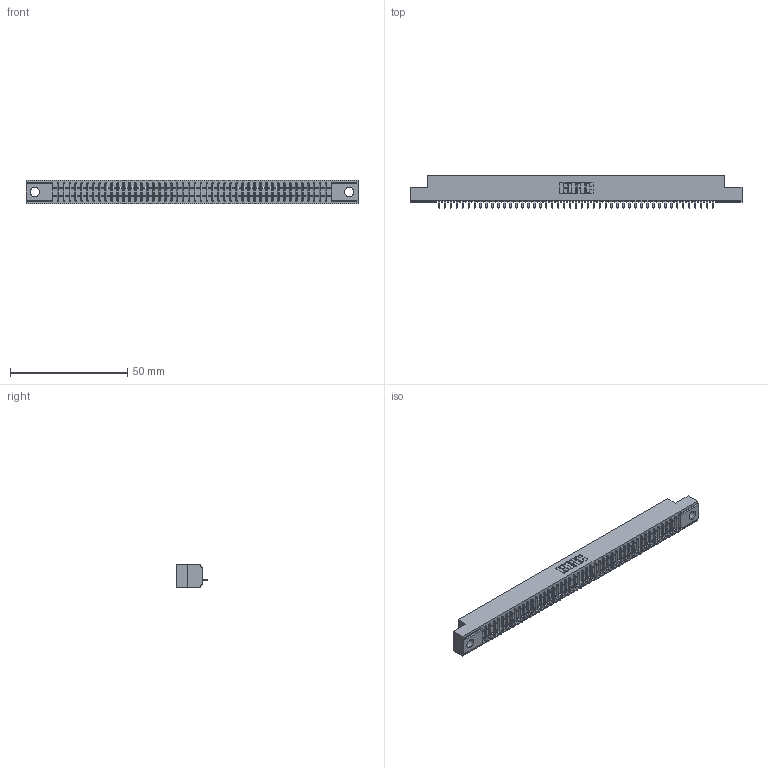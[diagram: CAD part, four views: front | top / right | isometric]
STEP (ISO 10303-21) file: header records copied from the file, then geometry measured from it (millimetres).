
FILE_DESCRIPTION (( 'STEP AP203' ), '1' );
FILE_NAME ('391-047-524-104.STEP', '2018-08-09T03:53:25', ( '' ), ( '' ), 'SwSTEP 2.0', 'SolidWorks 2016', '' );
FILE_SCHEMA (( 'CONFIG_CONTROL_DESIGN' ));
Length unit declared in the file: inch
Products named in the file (3): 341 Part_.156 (3.96) Dia Mounting Holes; 341-292-001_341-292-124; 391-047-524-104
Assembly tree (48 placements, depth 2):
  391-047-524-104
    341 Part_.156 (3.96) Dia Mounting Holes
    341-292-001_341-292-124  x47
Bounding box: 141.6 x 13.64 x 10.16 mm (x, y, z)
Volume: 10014.5 mm3; surface area: 15390.3 mm2
Topology: 48 solids, 48 shells, 3984 faces, 11491 edges, 7374 vertices
Faces by surface type: plane 2479, cylinder 1317, sphere 96, torus 92
Entity records: 55128 total; most frequent: CARTESIAN_POINT 9372, ORIENTED_EDGE 9358, DIRECTION 9035, EDGE_CURVE 4679, VECTOR 3793, LINE 3793, VERTEX_POINT 2958, AXIS2_PLACEMENT_3D 2621
